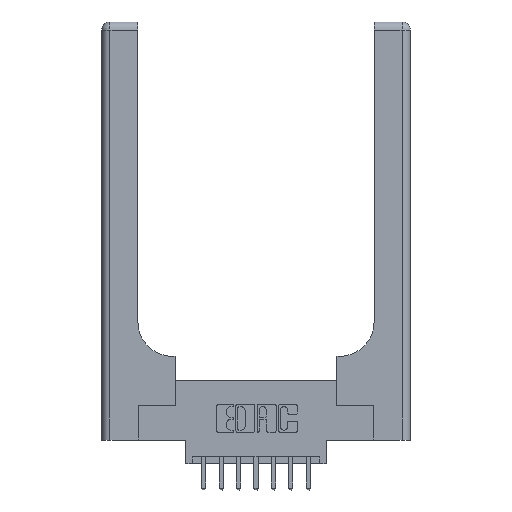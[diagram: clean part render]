
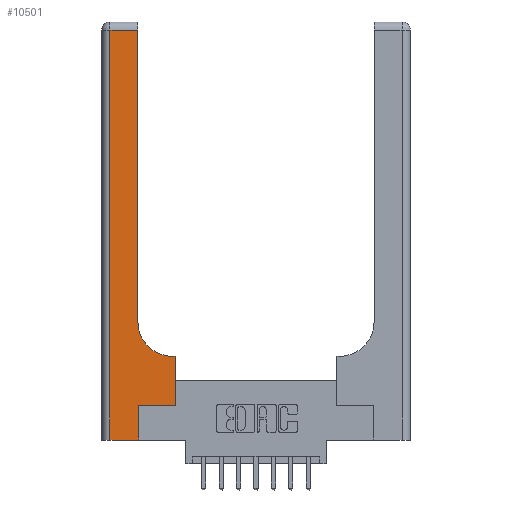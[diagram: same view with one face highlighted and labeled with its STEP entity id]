
A CAD part, top view. The second image highlights one B-rep face of the part: STEP entity #10501.
In plain terms, the highlighted planar face has unit normal (0, 0, 1).
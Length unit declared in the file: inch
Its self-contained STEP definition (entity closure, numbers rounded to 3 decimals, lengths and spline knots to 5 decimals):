
#16 = EDGE_LOOP ( 'NONE', ( #14900, #3506, #6034, #12678, #4338, #8928, #6045, #9793, #14614 ) ) ;
#26 = DIRECTION ( 'NONE',  ( 1., 0., 0. ) ) ;
#504 = EDGE_CURVE ( 'NONE', #14068, #10240, #14320, .T. ) ;
#609 = CARTESIAN_POINT ( 'NONE',  ( 0.06, 0., 0.37 ) ) ;
#875 = EDGE_CURVE ( 'NONE', #8678, #7442, #4785, .T. ) ;
#1060 = CARTESIAN_POINT ( 'NONE',  ( 0.265, 0., 0.37 ) ) ;
#1196 = CARTESIAN_POINT ( 'NONE',  ( 0.26, 3., 0.37 ) ) ;
#1461 = VECTOR ( 'NONE', #4799, 39.37008 ) ;
#1842 = AXIS2_PLACEMENT_3D ( 'NONE', #5779, #12847, #26 ) ;
#1896 = DIRECTION ( 'NONE',  ( 0., -1., 0. ) ) ;
#2072 = CARTESIAN_POINT ( 'NONE',  ( 0., 3., 0.37 ) ) ;
#2220 = DIRECTION ( 'NONE',  ( -1., 0., 0. ) ) ;
#2243 = DIRECTION ( 'NONE',  ( 0., 1., 0. ) ) ;
#2790 = DIRECTION ( 'NONE',  ( -1., 0., 0. ) ) ;
#2947 = VERTEX_POINT ( 'NONE', #9789 ) ;
#3219 = EDGE_CURVE ( 'NONE', #10240, #12719, #14453, .T. ) ;
#3441 = DIRECTION ( 'NONE',  ( 0., 0., -1. ) ) ;
#3506 = ORIENTED_EDGE ( 'NONE', *, *, #9202, .T. ) ;
#4269 = EDGE_CURVE ( 'NONE', #4302, #9533, #11554, .T. ) ;
#4302 = VERTEX_POINT ( 'NONE', #5413 ) ;
#4338 = ORIENTED_EDGE ( 'NONE', *, *, #4823, .T. ) ;
#4548 = AXIS2_PLACEMENT_3D ( 'NONE', #2072, #3441, #2220 ) ;
#4785 = LINE ( 'NONE', #1196, #6124 ) ;
#4799 = DIRECTION ( 'NONE',  ( 0., 1., 0. ) ) ;
#4823 = EDGE_CURVE ( 'NONE', #7887, #2947, #5777, .T. ) ;
#4974 = LINE ( 'NONE', #14485, #14782 ) ;
#5124 = DIRECTION ( 'NONE',  ( 1., 0., 0. ) ) ;
#5241 = CARTESIAN_POINT ( 'NONE',  ( 0.51, 0.6, 0.37 ) ) ;
#5313 = CARTESIAN_POINT ( 'NONE',  ( 0.26, 2.94, 0.37 ) ) ;
#5413 = CARTESIAN_POINT ( 'NONE',  ( 0.06, 2.94, 0.37 ) ) ;
#5598 = FACE_OUTER_BOUND ( 'NONE', #16, .T. ) ;
#5754 = PLANE ( 'NONE',  #4548 ) ;
#5777 = LINE ( 'NONE', #13983, #10101 ) ;
#5779 = CARTESIAN_POINT ( 'NONE',  ( 0.51, 0.85, 0.37 ) ) ;
#5858 = LINE ( 'NONE', #11547, #13089 ) ;
#5929 = VECTOR ( 'NONE', #1896, 39.37008 ) ;
#5992 = VECTOR ( 'NONE', #6831, 39.37008 ) ;
#6034 = ORIENTED_EDGE ( 'NONE', *, *, #4269, .T. ) ;
#6045 = ORIENTED_EDGE ( 'NONE', *, *, #504, .T. ) ;
#6124 = VECTOR ( 'NONE', #10774, 39.37008 ) ;
#6831 = DIRECTION ( 'NONE',  ( -1., 0., 0. ) ) ;
#6985 = LINE ( 'NONE', #7980, #5992 ) ;
#7442 = VERTEX_POINT ( 'NONE', #5313 ) ;
#7887 = VERTEX_POINT ( 'NONE', #1060 ) ;
#7980 = CARTESIAN_POINT ( 'NONE',  ( 0., 2.94, 0.37 ) ) ;
#8245 = EDGE_CURVE ( 'NONE', #9533, #7887, #5858, .T. ) ;
#8678 = VERTEX_POINT ( 'NONE', #12753 ) ;
#8768 = CARTESIAN_POINT ( 'NONE',  ( 0.26, 0.6, 0.37 ) ) ;
#8928 = ORIENTED_EDGE ( 'NONE', *, *, #12434, .T. ) ;
#9202 = EDGE_CURVE ( 'NONE', #7442, #4302, #6985, .T. ) ;
#9533 = VERTEX_POINT ( 'NONE', #609 ) ;
#9789 = CARTESIAN_POINT ( 'NONE',  ( 0.265, 0.25, 0.37 ) ) ;
#9793 = ORIENTED_EDGE ( 'NONE', *, *, #3219, .T. ) ;
#10101 = VECTOR ( 'NONE', #2243, 39.37008 ) ;
#10240 = VERTEX_POINT ( 'NONE', #14281 ) ;
#10501 = ADVANCED_FACE ( 'NONE', ( #5598 ), #5754, .F. ) ;
#10774 = DIRECTION ( 'NONE',  ( 0., 1., 0. ) ) ;
#11547 = CARTESIAN_POINT ( 'NONE',  ( 0., 0., 0.37 ) ) ;
#11554 = LINE ( 'NONE', #12709, #5929 ) ;
#12434 = EDGE_CURVE ( 'NONE', #2947, #14068, #4974, .T. ) ;
#12678 = ORIENTED_EDGE ( 'NONE', *, *, #8245, .T. ) ;
#12709 = CARTESIAN_POINT ( 'NONE',  ( 0.06, 3., 0.37 ) ) ;
#12719 = VERTEX_POINT ( 'NONE', #5241 ) ;
#12753 = CARTESIAN_POINT ( 'NONE',  ( 0.26, 0.85, 0.37 ) ) ;
#12847 = DIRECTION ( 'NONE',  ( 0., 0., -1. ) ) ;
#13089 = VECTOR ( 'NONE', #13853, 39.37008 ) ;
#13171 = CARTESIAN_POINT ( 'NONE',  ( 0.528, 0.25, 0.37 ) ) ;
#13587 = VECTOR ( 'NONE', #2790, 39.37008 ) ;
#13853 = DIRECTION ( 'NONE',  ( 1., 0., 0. ) ) ;
#13983 = CARTESIAN_POINT ( 'NONE',  ( 0.265, 0., 0.37 ) ) ;
#14001 = CARTESIAN_POINT ( 'NONE',  ( 0.528, 0.25, 0.37 ) ) ;
#14068 = VERTEX_POINT ( 'NONE', #14001 ) ;
#14281 = CARTESIAN_POINT ( 'NONE',  ( 0.528, 0.6, 0.37 ) ) ;
#14320 = LINE ( 'NONE', #13171, #1461 ) ;
#14453 = LINE ( 'NONE', #8768, #13587 ) ;
#14485 = CARTESIAN_POINT ( 'NONE',  ( 0.265, 0.25, 0.37 ) ) ;
#14545 = EDGE_CURVE ( 'NONE', #12719, #8678, #15073, .T. ) ;
#14614 = ORIENTED_EDGE ( 'NONE', *, *, #14545, .T. ) ;
#14782 = VECTOR ( 'NONE', #5124, 39.37008 ) ;
#14900 = ORIENTED_EDGE ( 'NONE', *, *, #875, .T. ) ;
#15073 = CIRCLE ( 'NONE', #1842, 0.25 ) ;
